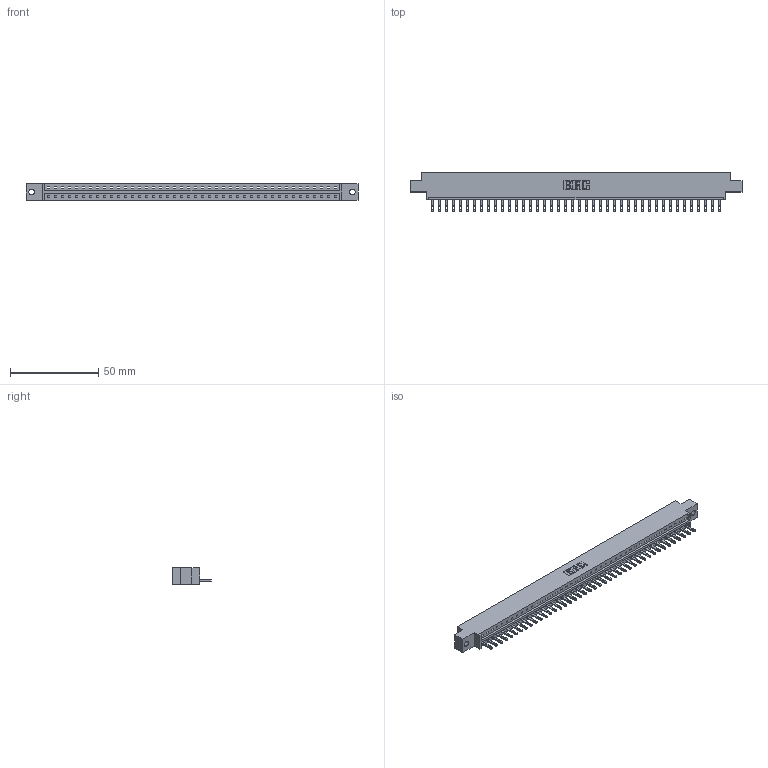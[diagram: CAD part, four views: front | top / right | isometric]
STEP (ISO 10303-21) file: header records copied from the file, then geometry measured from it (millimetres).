
FILE_DESCRIPTION (( 'STEP AP203' ), '1' );
FILE_NAME ('333-042-500-602.STEP', '2018-08-03T15:58:02', ( '' ), ( '' ), 'SwSTEP 2.0', 'SolidWorks 2016', '' );
FILE_SCHEMA (( 'CONFIG_CONTROL_DESIGN' ));
Length unit declared in the file: inch
Products named in the file (3): 345-292-001_345-293-100; 333-042-500-602; 333 Part_Offset - .128 Dia
Assembly tree (43 placements, depth 2):
  333-042-500-602
    333 Part_Offset - .128 Dia
    345-292-001_345-293-100  x42
Bounding box: 187.96 x 21.85 x 9.4 mm (x, y, z)
Volume: 18675.6 mm3; surface area: 20234.4 mm2
Topology: 43 solids, 43 shells, 2386 faces, 7379 edges, 4918 vertices
Faces by surface type: plane 1586, cylinder 800
Entity records: 25741 total; most frequent: CARTESIAN_POINT 4448, ORIENTED_EDGE 4426, DIRECTION 3753, EDGE_CURVE 2213, LINE 2081, VECTOR 2081, VERTEX_POINT 1474, AXIS2_PLACEMENT_3D 836
